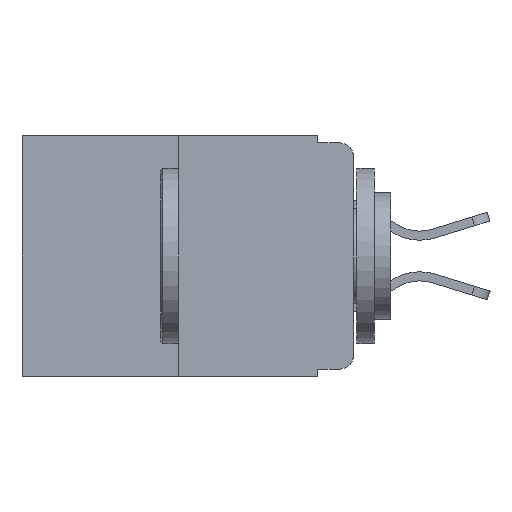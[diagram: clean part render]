
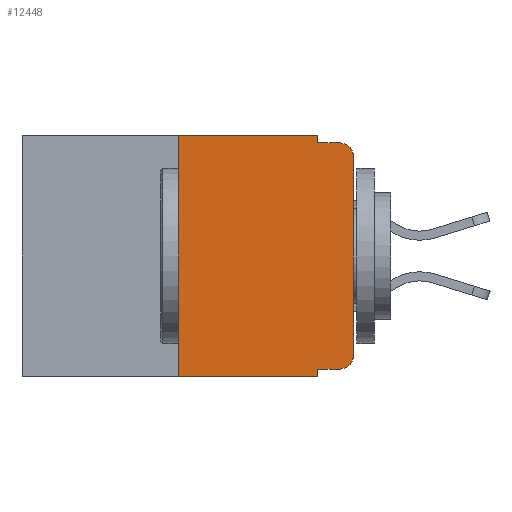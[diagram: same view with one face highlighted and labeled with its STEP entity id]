
A CAD part, left-side view. The second image highlights one B-rep face of the part: STEP entity #12448.
In plain terms, the highlighted planar face has unit normal (-1, 0, 0).
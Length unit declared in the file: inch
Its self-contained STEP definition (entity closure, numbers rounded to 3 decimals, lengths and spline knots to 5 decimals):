
#7 = CARTESIAN_POINT ( 'NONE',  ( 0., 0.051, -0.343 ) ) ;
#22 = DIRECTION ( 'NONE',  ( 0., 0., -1. ) ) ;
#323 = VECTOR ( 'NONE', #7828, 39.37008 ) ;
#341 = VECTOR ( 'NONE', #18717, 39.37008 ) ;
#430 = CARTESIAN_POINT ( 'NONE',  ( 0., 0.25, 0. ) ) ;
#696 = CARTESIAN_POINT ( 'NONE',  ( 0., 0., 0. ) ) ;
#1474 = VERTEX_POINT ( 'NONE', #7783 ) ;
#1760 = CARTESIAN_POINT ( 'NONE',  ( 0., 0.02, -0.01 ) ) ;
#1816 = CARTESIAN_POINT ( 'NONE',  ( 0., 0.473, -0.343 ) ) ;
#1833 = ORIENTED_EDGE ( 'NONE', *, *, #11556, .T. ) ;
#2934 = EDGE_CURVE ( 'NONE', #7461, #2963, #4649, .T. ) ;
#2963 = VERTEX_POINT ( 'NONE', #12091 ) ;
#3083 = VERTEX_POINT ( 'NONE', #1760 ) ;
#3313 = VECTOR ( 'NONE', #17887, 39.37008 ) ;
#3561 = EDGE_CURVE ( 'NONE', #7275, #12052, #6277, .T. ) ;
#4129 = VECTOR ( 'NONE', #6947, 39.37008 ) ;
#4351 = VECTOR ( 'NONE', #19817, 39.37008 ) ;
#4649 = LINE ( 'NONE', #14735, #14981 ) ;
#5010 = DIRECTION ( 'NONE',  ( 1., 0., 0. ) ) ;
#5296 = CARTESIAN_POINT ( 'NONE',  ( 0., 0.25, 0. ) ) ;
#6239 = DIRECTION ( 'NONE',  ( -1., 0., 0. ) ) ;
#6277 = CIRCLE ( 'NONE', #12077, 0.02 ) ;
#6696 = EDGE_CURVE ( 'NONE', #1474, #7461, #21221, .T. ) ;
#6947 = DIRECTION ( 'NONE',  ( 0., -1., 0. ) ) ;
#7275 = VERTEX_POINT ( 'NONE', #20383 ) ;
#7461 = VERTEX_POINT ( 'NONE', #5296 ) ;
#7783 = CARTESIAN_POINT ( 'NONE',  ( 0., 0.25, -0.343 ) ) ;
#7828 = DIRECTION ( 'NONE',  ( 0., 0., 1. ) ) ;
#7905 = ORIENTED_EDGE ( 'NONE', *, *, #3561, .T. ) ;
#8081 = ORIENTED_EDGE ( 'NONE', *, *, #8148, .T. ) ;
#8148 = EDGE_CURVE ( 'NONE', #16049, #3083, #18985, .T. ) ;
#8640 = ORIENTED_EDGE ( 'NONE', *, *, #16489, .T. ) ;
#8729 = ORIENTED_EDGE ( 'NONE', *, *, #2934, .F. ) ;
#9039 = ORIENTED_EDGE ( 'NONE', *, *, #6696, .F. ) ;
#9651 = DIRECTION ( 'NONE',  ( 0., 0., -1. ) ) ;
#10116 = DIRECTION ( 'NONE',  ( 0., 0., -1. ) ) ;
#10371 = LINE ( 'NONE', #12075, #17433 ) ;
#11233 = EDGE_CURVE ( 'NONE', #2963, #11760, #18826, .T. ) ;
#11355 = CARTESIAN_POINT ( 'NONE',  ( 0., 0.02, -0.03 ) ) ;
#11556 = EDGE_CURVE ( 'NONE', #19490, #7275, #16403, .T. ) ;
#11715 = CARTESIAN_POINT ( 'NONE',  ( 0., 0.473, 0. ) ) ;
#11760 = VERTEX_POINT ( 'NONE', #22204 ) ;
#12052 = VERTEX_POINT ( 'NONE', #15137 ) ;
#12075 = CARTESIAN_POINT ( 'NONE',  ( 0., 0.051, 0. ) ) ;
#12077 = AXIS2_PLACEMENT_3D ( 'NONE', #13857, #15680, #12288 ) ;
#12091 = CARTESIAN_POINT ( 'NONE',  ( 0., 0.051, 0. ) ) ;
#12288 = DIRECTION ( 'NONE',  ( 0., 0., -1. ) ) ;
#12448 = ADVANCED_FACE ( 'NONE', ( #15441 ), #16703, .F. ) ;
#12850 = DIRECTION ( 'NONE',  ( 0., 0., 1. ) ) ;
#13344 = EDGE_CURVE ( 'NONE', #19490, #13686, #10371, .T. ) ;
#13686 = VERTEX_POINT ( 'NONE', #7 ) ;
#13739 = CARTESIAN_POINT ( 'NONE',  ( 0., 0.051, -0.01 ) ) ;
#13806 = ORIENTED_EDGE ( 'NONE', *, *, #11233, .F. ) ;
#13857 = CARTESIAN_POINT ( 'NONE',  ( 0., 0.02, -0.313 ) ) ;
#13921 = CARTESIAN_POINT ( 'NONE',  ( 0., 0.051, 0. ) ) ;
#14266 = EDGE_CURVE ( 'NONE', #1474, #13686, #20765, .T. ) ;
#14735 = CARTESIAN_POINT ( 'NONE',  ( 0., 0.473, 0. ) ) ;
#14981 = VECTOR ( 'NONE', #18265, 39.37008 ) ;
#15137 = CARTESIAN_POINT ( 'NONE',  ( 0., 0., -0.313 ) ) ;
#15441 = FACE_OUTER_BOUND ( 'NONE', #16460, .T. ) ;
#15680 = DIRECTION ( 'NONE',  ( -1., 0., 0. ) ) ;
#15761 = ORIENTED_EDGE ( 'NONE', *, *, #16727, .F. ) ;
#16049 = VERTEX_POINT ( 'NONE', #19167 ) ;
#16249 = LINE ( 'NONE', #696, #18282 ) ;
#16403 = LINE ( 'NONE', #21985, #4351 ) ;
#16460 = EDGE_LOOP ( 'NONE', ( #8640, #8081, #15761, #13806, #8729, #9039, #22031, #21424, #1833, #7905 ) ) ;
#16489 = EDGE_CURVE ( 'NONE', #12052, #16049, #16249, .T. ) ;
#16703 = PLANE ( 'NONE',  #18097 ) ;
#16727 = EDGE_CURVE ( 'NONE', #11760, #3083, #17042, .T. ) ;
#17042 = LINE ( 'NONE', #13739, #4129 ) ;
#17433 = VECTOR ( 'NONE', #22, 39.37008 ) ;
#17887 = DIRECTION ( 'NONE',  ( 0., -1., 0. ) ) ;
#18097 = AXIS2_PLACEMENT_3D ( 'NONE', #11715, #5010, #10116 ) ;
#18265 = DIRECTION ( 'NONE',  ( 0., -1., 0. ) ) ;
#18282 = VECTOR ( 'NONE', #12850, 39.37008 ) ;
#18717 = DIRECTION ( 'NONE',  ( 0., 0., -1. ) ) ;
#18826 = LINE ( 'NONE', #13921, #341 ) ;
#18985 = CIRCLE ( 'NONE', #21889, 0.02 ) ;
#19167 = CARTESIAN_POINT ( 'NONE',  ( 0., 0., -0.03 ) ) ;
#19490 = VERTEX_POINT ( 'NONE', #21695 ) ;
#19817 = DIRECTION ( 'NONE',  ( 0., -1., 0. ) ) ;
#20383 = CARTESIAN_POINT ( 'NONE',  ( 0., 0.02, -0.333 ) ) ;
#20765 = LINE ( 'NONE', #1816, #3313 ) ;
#21221 = LINE ( 'NONE', #430, #323 ) ;
#21424 = ORIENTED_EDGE ( 'NONE', *, *, #13344, .F. ) ;
#21695 = CARTESIAN_POINT ( 'NONE',  ( 0., 0.051, -0.333 ) ) ;
#21889 = AXIS2_PLACEMENT_3D ( 'NONE', #11355, #6239, #9651 ) ;
#21985 = CARTESIAN_POINT ( 'NONE',  ( 0., 0.051, -0.333 ) ) ;
#22031 = ORIENTED_EDGE ( 'NONE', *, *, #14266, .T. ) ;
#22204 = CARTESIAN_POINT ( 'NONE',  ( 0., 0.051, -0.01 ) ) ;
